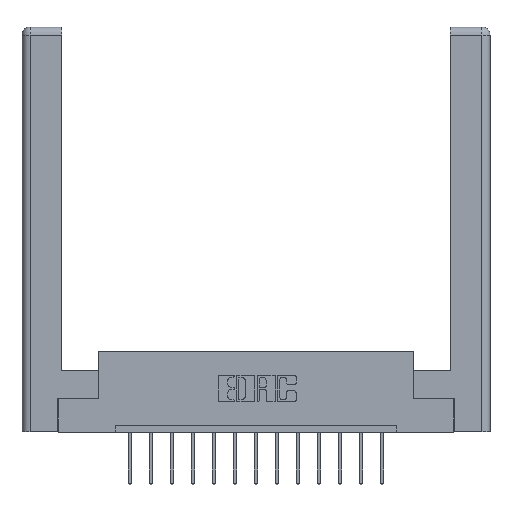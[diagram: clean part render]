
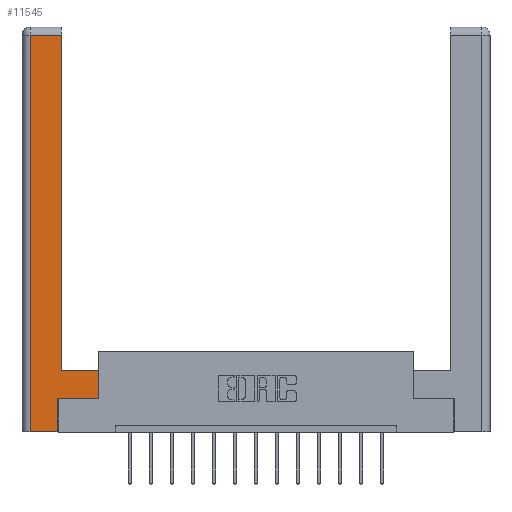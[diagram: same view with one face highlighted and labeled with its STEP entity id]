
A CAD part, top view. The second image highlights one B-rep face of the part: STEP entity #11545.
In plain terms, the highlighted planar face has unit normal (0, 0, 1).
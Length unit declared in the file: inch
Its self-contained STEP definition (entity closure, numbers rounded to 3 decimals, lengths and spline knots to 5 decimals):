
#157 = VERTEX_POINT ( 'NONE', #3946 ) ;
#297 = DIRECTION ( 'NONE',  ( -1., 0., 0. ) ) ;
#435 = LINE ( 'NONE', #9930, #13214 ) ;
#1031 = DIRECTION ( 'NONE',  ( 0., 1., 0. ) ) ;
#1089 = ORIENTED_EDGE ( 'NONE', *, *, #12463, .T. ) ;
#1327 = DIRECTION ( 'NONE',  ( 0., 1., 0. ) ) ;
#1457 = VERTEX_POINT ( 'NONE', #6809 ) ;
#1654 = VECTOR ( 'NONE', #3546, 39.37008 ) ;
#1661 = VERTEX_POINT ( 'NONE', #2973 ) ;
#1832 = EDGE_CURVE ( 'NONE', #1457, #12979, #8084, .T. ) ;
#2050 = DIRECTION ( 'NONE',  ( -1., 0., 0. ) ) ;
#2266 = ORIENTED_EDGE ( 'NONE', *, *, #3911, .T. ) ;
#2313 = VERTEX_POINT ( 'NONE', #5587 ) ;
#2694 = VECTOR ( 'NONE', #297, 39.37008 ) ;
#2829 = CARTESIAN_POINT ( 'NONE',  ( 0.0615, 2.94, 0. ) ) ;
#2973 = CARTESIAN_POINT ( 'NONE',  ( 0.565, 0.245, 0. ) ) ;
#3101 = CARTESIAN_POINT ( 'NONE',  ( 0.265, 0.245, 0. ) ) ;
#3392 = EDGE_CURVE ( 'NONE', #1661, #1457, #4511, .T. ) ;
#3546 = DIRECTION ( 'NONE',  ( 1., 0., 0. ) ) ;
#3911 = EDGE_CURVE ( 'NONE', #12979, #10034, #435, .T. ) ;
#3946 = CARTESIAN_POINT ( 'NONE',  ( 0.0615, 0., 0. ) ) ;
#4068 = LINE ( 'NONE', #6028, #13556 ) ;
#4111 = ORIENTED_EDGE ( 'NONE', *, *, #3392, .T. ) ;
#4279 = EDGE_LOOP ( 'NONE', ( #2266, #1089, #14823, #12933, #13291, #6005, #4111, #11864 ) ) ;
#4511 = LINE ( 'NONE', #8582, #13627 ) ;
#4703 = EDGE_CURVE ( 'NONE', #2313, #15560, #11469, .T. ) ;
#4805 = VERTEX_POINT ( 'NONE', #11110 ) ;
#4826 = DIRECTION ( 'NONE',  ( 1., 0., 0. ) ) ;
#5131 = DIRECTION ( 'NONE',  ( 0., 0., -1. ) ) ;
#5447 = CARTESIAN_POINT ( 'NONE',  ( 0.295, 0.45, 0. ) ) ;
#5587 = CARTESIAN_POINT ( 'NONE',  ( 0.265, 0., 0. ) ) ;
#5654 = EDGE_CURVE ( 'NONE', #15560, #1661, #4068, .T. ) ;
#6005 = ORIENTED_EDGE ( 'NONE', *, *, #5654, .T. ) ;
#6028 = CARTESIAN_POINT ( 'NONE',  ( 0.565, 0.245, 0. ) ) ;
#6187 = EDGE_CURVE ( 'NONE', #157, #2313, #12329, .T. ) ;
#6191 = DIRECTION ( 'NONE',  ( -1., 0., 0. ) ) ;
#6273 = CARTESIAN_POINT ( 'NONE',  ( 0.295, 2.94, 0. ) ) ;
#6425 = VECTOR ( 'NONE', #15791, 39.37008 ) ;
#6517 = VECTOR ( 'NONE', #2050, 39.37008 ) ;
#6809 = CARTESIAN_POINT ( 'NONE',  ( 0.565, 0.45, 0. ) ) ;
#8084 = LINE ( 'NONE', #11747, #6517 ) ;
#8582 = CARTESIAN_POINT ( 'NONE',  ( 0.565, 0.45, 0. ) ) ;
#8616 = DIRECTION ( 'NONE',  ( 0., -1., 0. ) ) ;
#8872 = VECTOR ( 'NONE', #8616, 39.37008 ) ;
#9608 = LINE ( 'NONE', #11165, #8872 ) ;
#9930 = CARTESIAN_POINT ( 'NONE',  ( 0.295, 3., 0. ) ) ;
#10020 = CARTESIAN_POINT ( 'NONE',  ( 0., 0., 0. ) ) ;
#10034 = VERTEX_POINT ( 'NONE', #6273 ) ;
#10246 = AXIS2_PLACEMENT_3D ( 'NONE', #10020, #5131, #6191 ) ;
#10727 = CARTESIAN_POINT ( 'NONE',  ( 0.265, 0.245, 0. ) ) ;
#11110 = CARTESIAN_POINT ( 'NONE',  ( 0.0615, 2.94, 0. ) ) ;
#11165 = CARTESIAN_POINT ( 'NONE',  ( 0.0615, 0., 0. ) ) ;
#11469 = LINE ( 'NONE', #10727, #6425 ) ;
#11545 = ADVANCED_FACE ( 'NONE', ( #11778 ), #14482, .F. ) ;
#11747 = CARTESIAN_POINT ( 'NONE',  ( 0.295, 0.45, 0. ) ) ;
#11778 = FACE_OUTER_BOUND ( 'NONE', #4279, .T. ) ;
#11864 = ORIENTED_EDGE ( 'NONE', *, *, #1832, .T. ) ;
#12261 = CARTESIAN_POINT ( 'NONE',  ( 0.265, 0., 0. ) ) ;
#12329 = LINE ( 'NONE', #12261, #1654 ) ;
#12463 = EDGE_CURVE ( 'NONE', #10034, #4805, #13755, .T. ) ;
#12933 = ORIENTED_EDGE ( 'NONE', *, *, #6187, .T. ) ;
#12979 = VERTEX_POINT ( 'NONE', #5447 ) ;
#13214 = VECTOR ( 'NONE', #1327, 39.37008 ) ;
#13291 = ORIENTED_EDGE ( 'NONE', *, *, #4703, .T. ) ;
#13556 = VECTOR ( 'NONE', #4826, 39.37008 ) ;
#13627 = VECTOR ( 'NONE', #1031, 39.37008 ) ;
#13755 = LINE ( 'NONE', #2829, #2694 ) ;
#13760 = EDGE_CURVE ( 'NONE', #4805, #157, #9608, .T. ) ;
#14482 = PLANE ( 'NONE',  #10246 ) ;
#14823 = ORIENTED_EDGE ( 'NONE', *, *, #13760, .T. ) ;
#15560 = VERTEX_POINT ( 'NONE', #3101 ) ;
#15791 = DIRECTION ( 'NONE',  ( 0., 1., 0. ) ) ;
